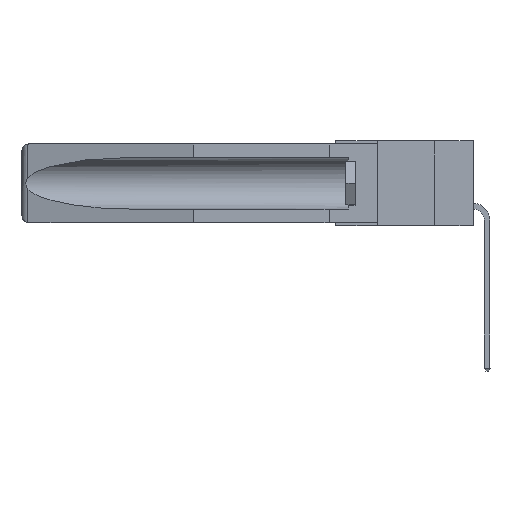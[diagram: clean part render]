
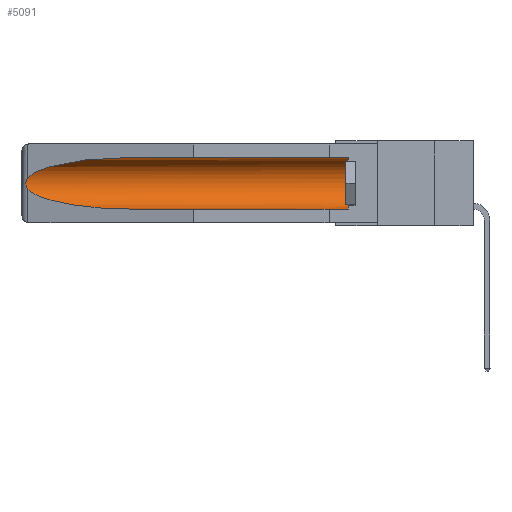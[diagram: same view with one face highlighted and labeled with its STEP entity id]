
A CAD part, left-side view. The second image highlights one B-rep face of the part: STEP entity #5091.
In plain terms, the highlighted cylindrical face has radius 2.857 mm (diameter 5.715 mm), a partial arc.
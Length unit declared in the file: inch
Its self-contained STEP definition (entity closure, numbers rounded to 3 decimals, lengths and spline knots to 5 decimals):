
#69 = VERTEX_POINT ( 'NONE', #15942 ) ;
#615 = CARTESIAN_POINT ( 'NONE',  ( 0.155, 0.126, -0.1715 ) ) ;
#1435 = ORIENTED_EDGE ( 'NONE', *, *, #15434, .T. ) ;
#2283 = CIRCLE ( 'NONE', #17850, 0.1125 ) ;
#2479 = EDGE_CURVE ( 'NONE', #23355, #21892, #2963, .T. ) ;
#2963 =( BOUNDED_CURVE ( )  B_SPLINE_CURVE ( 3, ( #8471, #23094, #6585, #16236 ),
 .UNSPECIFIED., .F., .F. ) 
 B_SPLINE_CURVE_WITH_KNOTS ( ( 4, 4 ),
 ( 0.1948, 1.5708 ),
 .UNSPECIFIED. ) 
 CURVE ( )  GEOMETRIC_REPRESENTATION_ITEM ( )  RATIONAL_B_SPLINE_CURVE ( ( 1., 0.848, 0.848, 1. ) ) 
 REPRESENTATION_ITEM ( '' )  );
#2999 = CARTESIAN_POINT ( 'NONE',  ( 0.21114, 1.30732, -0.059 ) ) ;
#3152 = DIRECTION ( 'NONE',  ( 0., 1., 0. ) ) ;
#3164 = LINE ( 'NONE', #26083, #5440 ) ;
#3597 = EDGE_CURVE ( 'NONE', #20541, #69, #27088, .T. ) ;
#4375 = EDGE_CURVE ( 'NONE', #69, #23355, #19682, .T. ) ;
#4473 = CARTESIAN_POINT ( 'NONE',  ( 0.155, 0.126, -0.059 ) ) ;
#4802 = DIRECTION ( 'NONE',  ( 0., 1., 0. ) ) ;
#4865 = VERTEX_POINT ( 'NONE', #15559 ) ;
#5091 = ADVANCED_FACE ( 'NONE', ( #8058 ), #23440, .F. ) ;
#5219 = CARTESIAN_POINT ( 'NONE',  ( 0.2673, 1.53269, -0.17917 ) ) ;
#5356 = CARTESIAN_POINT ( 'NONE',  ( 0.155, 1.07973, -0.059 ) ) ;
#5396 = CARTESIAN_POINT ( 'NONE',  ( 0.2673, 1.5327, -0.16383 ) ) ;
#5440 = VECTOR ( 'NONE', #3152, 39.37008 ) ;
#5543 = CARTESIAN_POINT ( 'NONE',  ( 0.155, 1.07973, -0.059 ) ) ;
#6079 = ORIENTED_EDGE ( 'NONE', *, *, #4375, .T. ) ;
#6096 = ORIENTED_EDGE ( 'NONE', *, *, #2479, .T. ) ;
#6585 = CARTESIAN_POINT ( 'NONE',  ( 0.21114, 1.30732, -0.284 ) ) ;
#6929 = DIRECTION ( 'NONE',  ( 0., -1., 0. ) ) ;
#7312 = CARTESIAN_POINT ( 'NONE',  ( 0.26655, 1.53094, -0.18657 ) ) ;
#8037 = ORIENTED_EDGE ( 'NONE', *, *, #20047, .F. ) ;
#8058 = FACE_OUTER_BOUND ( 'NONE', #13465, .T. ) ;
#8077 = ORIENTED_EDGE ( 'NONE', *, *, #3597, .T. ) ;
#8471 = CARTESIAN_POINT ( 'NONE',  ( 0.26537, 1.52718, -0.19328 ) ) ;
#8763 = DIRECTION ( 'NONE',  ( 0., 0., 1. ) ) ;
#8871 = CARTESIAN_POINT ( 'NONE',  ( 0.26537, 1.52718, -0.14972 ) ) ;
#9452 = CARTESIAN_POINT ( 'NONE',  ( 0.2675, 1.53308, -0.16763 ) ) ;
#10491 = CARTESIAN_POINT ( 'NONE',  ( 0.26537, 1.52718, -0.19328 ) ) ;
#11249 = CARTESIAN_POINT ( 'NONE',  ( 0.155, -0.30754, -0.059 ) ) ;
#11544 = CARTESIAN_POINT ( 'NONE',  ( 0.25451, 1.48313, -0.09465 ) ) ;
#12749 = VECTOR ( 'NONE', #4802, 39.37008 ) ;
#13465 = EDGE_LOOP ( 'NONE', ( #8077, #6079, #6096, #8037, #25790, #1435 ) ) ;
#15132 = CARTESIAN_POINT ( 'NONE',  ( 0.155, -0.30754, -0.1715 ) ) ;
#15406 = LINE ( 'NONE', #11249, #12749 ) ;
#15434 = EDGE_CURVE ( 'NONE', #15740, #20541, #15406, .T. ) ;
#15559 = CARTESIAN_POINT ( 'NONE',  ( 0.155, 0.126, -0.284 ) ) ;
#15740 = VERTEX_POINT ( 'NONE', #4473 ) ;
#15942 = CARTESIAN_POINT ( 'NONE',  ( 0.26537, 1.52718, -0.14972 ) ) ;
#16236 = CARTESIAN_POINT ( 'NONE',  ( 0.155, 1.07973, -0.284 ) ) ;
#17850 = AXIS2_PLACEMENT_3D ( 'NONE', #615, #6929, #8763 ) ;
#18006 = EDGE_CURVE ( 'NONE', #4865, #15740, #2283, .T. ) ;
#19682 = B_SPLINE_CURVE_WITH_KNOTS ( 'NONE', 3,
 ( #8871, #25433, #25881, #5396, #9452, #19920, #5219, #7312, #21930, #21662 ),
 .UNSPECIFIED., .F., .F.,
 ( 4, 2, 2, 2, 4 ),
 ( 0., 0.00029, 0.00058, 0.00087, 0.00117 ),
 .UNSPECIFIED. ) ;
#19920 = CARTESIAN_POINT ( 'NONE',  ( 0.2675, 1.53308, -0.17534 ) ) ;
#20047 = EDGE_CURVE ( 'NONE', #4865, #21892, #3164, .T. ) ;
#20519 = AXIS2_PLACEMENT_3D ( 'NONE', #15132, #21347, #23518 ) ;
#20541 = VERTEX_POINT ( 'NONE', #5543 ) ;
#21347 = DIRECTION ( 'NONE',  ( 0., 1., 0. ) ) ;
#21662 = CARTESIAN_POINT ( 'NONE',  ( 0.26537, 1.52718, -0.19328 ) ) ;
#21892 = VERTEX_POINT ( 'NONE', #25185 ) ;
#21930 = CARTESIAN_POINT ( 'NONE',  ( 0.26597, 1.5296, -0.19026 ) ) ;
#23094 = CARTESIAN_POINT ( 'NONE',  ( 0.25451, 1.48313, -0.24835 ) ) ;
#23355 = VERTEX_POINT ( 'NONE', #10491 ) ;
#23440 = CYLINDRICAL_SURFACE ( 'NONE', #20519, 0.1125 ) ;
#23518 = DIRECTION ( 'NONE',  ( 0., 0., 1. ) ) ;
#24068 = CARTESIAN_POINT ( 'NONE',  ( 0.26537, 1.52718, -0.14972 ) ) ;
#25185 = CARTESIAN_POINT ( 'NONE',  ( 0.155, 1.07973, -0.284 ) ) ;
#25433 = CARTESIAN_POINT ( 'NONE',  ( 0.26597, 1.52961, -0.15275 ) ) ;
#25790 = ORIENTED_EDGE ( 'NONE', *, *, #18006, .T. ) ;
#25881 = CARTESIAN_POINT ( 'NONE',  ( 0.26654, 1.53092, -0.15636 ) ) ;
#26083 = CARTESIAN_POINT ( 'NONE',  ( 0.155, -0.30754, -0.284 ) ) ;
#27088 =( BOUNDED_CURVE ( )  B_SPLINE_CURVE ( 3, ( #5356, #2999, #11544, #24068 ),
 .UNSPECIFIED., .F., .T. ) 
 B_SPLINE_CURVE_WITH_KNOTS ( ( 4, 4 ),
 ( 4.71239, 6.08839 ),
 .UNSPECIFIED. ) 
 CURVE ( )  GEOMETRIC_REPRESENTATION_ITEM ( )  RATIONAL_B_SPLINE_CURVE ( ( 1., 0.848, 0.848, 1. ) ) 
 REPRESENTATION_ITEM ( '' )  );
